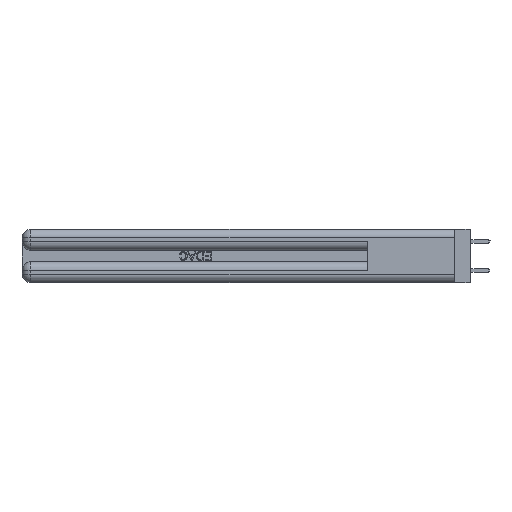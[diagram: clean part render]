
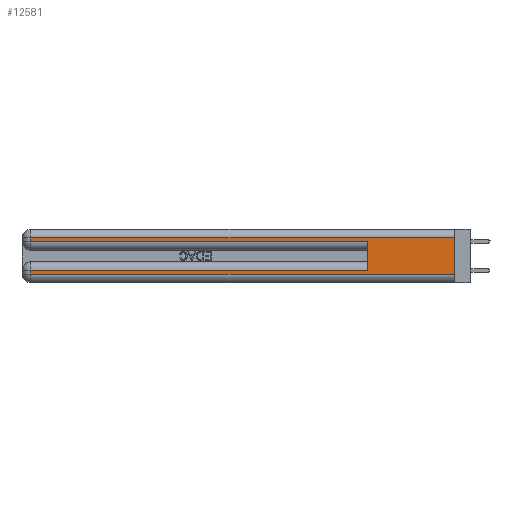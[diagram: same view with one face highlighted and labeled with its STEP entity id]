
A CAD part, left-side view. The second image highlights one B-rep face of the part: STEP entity #12581.
In plain terms, the highlighted planar face has unit normal (-1, 0, 0).
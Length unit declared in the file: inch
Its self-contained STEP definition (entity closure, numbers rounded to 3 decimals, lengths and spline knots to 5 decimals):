
#518 = LINE ( 'NONE', #14102, #24356 ) ;
#894 = DIRECTION ( 'NONE',  ( 1., 0., 0. ) ) ;
#942 = CARTESIAN_POINT ( 'NONE',  ( 0., 2.94, 0.085 ) ) ;
#1293 = DIRECTION ( 'NONE',  ( 0., 1., 0. ) ) ;
#2604 = VECTOR ( 'NONE', #28425, 39.37008 ) ;
#2826 = CARTESIAN_POINT ( 'NONE',  ( 0., 2.94, 0.37 ) ) ;
#3687 = EDGE_CURVE ( 'NONE', #22863, #35686, #518, .T. ) ;
#4988 = PLANE ( 'NONE',  #16196 ) ;
#5720 = CARTESIAN_POINT ( 'NONE',  ( 0., 0.6, 0.085 ) ) ;
#6030 = CARTESIAN_POINT ( 'NONE',  ( 0., 0.6, 0.145 ) ) ;
#7678 = EDGE_CURVE ( 'NONE', #10859, #40256, #17726, .T. ) ;
#8620 = EDGE_CURVE ( 'NONE', #27456, #21181, #15296, .T. ) ;
#9090 = EDGE_LOOP ( 'NONE', ( #40535, #31409, #31785, #33505, #28337, #25077, #42972, #45879 ) ) ;
#10859 = VERTEX_POINT ( 'NONE', #5720 ) ;
#11616 = VECTOR ( 'NONE', #24323, 39.37008 ) ;
#12581 = ADVANCED_FACE ( 'NONE', ( #31200 ), #4988, .F. ) ;
#13141 = LINE ( 'NONE', #2826, #47383 ) ;
#13655 = LINE ( 'NONE', #39362, #2604 ) ;
#14102 = CARTESIAN_POINT ( 'NONE',  ( 0., 0., 0.06 ) ) ;
#15296 = LINE ( 'NONE', #31209, #45410 ) ;
#16196 = AXIS2_PLACEMENT_3D ( 'NONE', #19849, #894, #26934 ) ;
#17044 = EDGE_CURVE ( 'NONE', #40256, #22863, #13141, .T. ) ;
#17726 = LINE ( 'NONE', #26130, #31666 ) ;
#19849 = CARTESIAN_POINT ( 'NONE',  ( 0., 0., 0.37 ) ) ;
#20659 = CARTESIAN_POINT ( 'NONE',  ( 0., 0., 0.06 ) ) ;
#21181 = VERTEX_POINT ( 'NONE', #43521 ) ;
#22863 = VERTEX_POINT ( 'NONE', #27035 ) ;
#23128 = VERTEX_POINT ( 'NONE', #43992 ) ;
#23492 = EDGE_CURVE ( 'NONE', #27456, #35686, #45614, .T. ) ;
#23553 = CARTESIAN_POINT ( 'NONE',  ( 0., 0., 0.37 ) ) ;
#24323 = DIRECTION ( 'NONE',  ( 0., 0., 1. ) ) ;
#24356 = VECTOR ( 'NONE', #43702, 39.37008 ) ;
#25077 = ORIENTED_EDGE ( 'NONE', *, *, #7678, .T. ) ;
#25849 = DIRECTION ( 'NONE',  ( 0., 0., -1. ) ) ;
#26130 = CARTESIAN_POINT ( 'NONE',  ( 0., 0., 0.085 ) ) ;
#26534 = CARTESIAN_POINT ( 'NONE',  ( 0., 2.94, 0.37 ) ) ;
#26934 = DIRECTION ( 'NONE',  ( 0., 0., -1. ) ) ;
#27035 = CARTESIAN_POINT ( 'NONE',  ( 0., 2.94, 0.06 ) ) ;
#27456 = VERTEX_POINT ( 'NONE', #34883 ) ;
#27861 = LINE ( 'NONE', #6030, #11616 ) ;
#28337 = ORIENTED_EDGE ( 'NONE', *, *, #44218, .F. ) ;
#28425 = DIRECTION ( 'NONE',  ( 0., -1., 0. ) ) ;
#31085 = DIRECTION ( 'NONE',  ( 0., 0., -1. ) ) ;
#31200 = FACE_OUTER_BOUND ( 'NONE', #9090, .T. ) ;
#31209 = CARTESIAN_POINT ( 'NONE',  ( 0., 0., 0.31 ) ) ;
#31263 = EDGE_CURVE ( 'NONE', #23128, #37733, #13655, .T. ) ;
#31409 = ORIENTED_EDGE ( 'NONE', *, *, #8620, .T. ) ;
#31666 = VECTOR ( 'NONE', #42598, 39.37008 ) ;
#31785 = ORIENTED_EDGE ( 'NONE', *, *, #37191, .T. ) ;
#33505 = ORIENTED_EDGE ( 'NONE', *, *, #31263, .T. ) ;
#34883 = CARTESIAN_POINT ( 'NONE',  ( 0., 0., 0.31 ) ) ;
#35686 = VERTEX_POINT ( 'NONE', #20659 ) ;
#35787 = VECTOR ( 'NONE', #45918, 39.37008 ) ;
#36683 = CARTESIAN_POINT ( 'NONE',  ( 0., 0.6, 0.285 ) ) ;
#37191 = EDGE_CURVE ( 'NONE', #21181, #23128, #41263, .T. ) ;
#37733 = VERTEX_POINT ( 'NONE', #36683 ) ;
#39362 = CARTESIAN_POINT ( 'NONE',  ( 0., 0., 0.285 ) ) ;
#40256 = VERTEX_POINT ( 'NONE', #942 ) ;
#40535 = ORIENTED_EDGE ( 'NONE', *, *, #23492, .F. ) ;
#41263 = LINE ( 'NONE', #26534, #47699 ) ;
#42598 = DIRECTION ( 'NONE',  ( 0., 1., 0. ) ) ;
#42972 = ORIENTED_EDGE ( 'NONE', *, *, #17044, .T. ) ;
#43521 = CARTESIAN_POINT ( 'NONE',  ( 0., 2.94, 0.31 ) ) ;
#43702 = DIRECTION ( 'NONE',  ( 0., -1., 0. ) ) ;
#43992 = CARTESIAN_POINT ( 'NONE',  ( 0., 2.94, 0.285 ) ) ;
#44218 = EDGE_CURVE ( 'NONE', #10859, #37733, #27861, .T. ) ;
#45410 = VECTOR ( 'NONE', #1293, 39.37008 ) ;
#45614 = LINE ( 'NONE', #23553, #35787 ) ;
#45879 = ORIENTED_EDGE ( 'NONE', *, *, #3687, .T. ) ;
#45918 = DIRECTION ( 'NONE',  ( 0., 0., -1. ) ) ;
#47383 = VECTOR ( 'NONE', #25849, 39.37008 ) ;
#47699 = VECTOR ( 'NONE', #31085, 39.37008 ) ;
